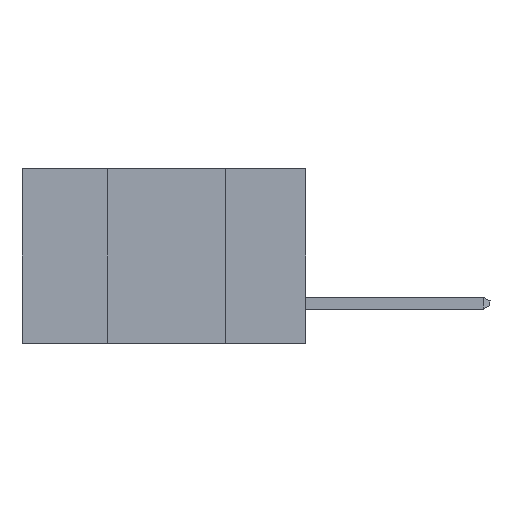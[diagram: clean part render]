
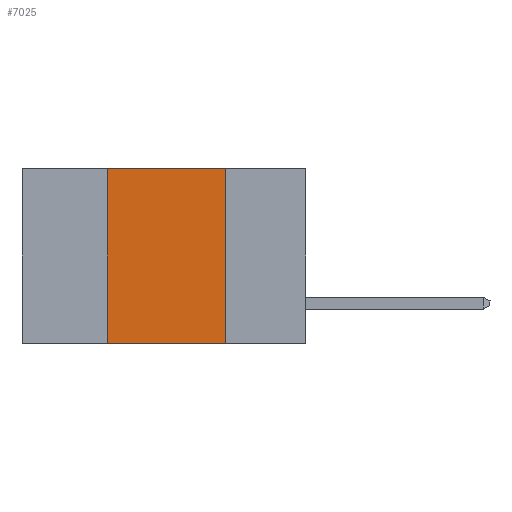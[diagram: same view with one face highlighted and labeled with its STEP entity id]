
A CAD part, left-side view. The second image highlights one B-rep face of the part: STEP entity #7025.
In plain terms, the highlighted planar face has unit normal (-1, 0, 0).
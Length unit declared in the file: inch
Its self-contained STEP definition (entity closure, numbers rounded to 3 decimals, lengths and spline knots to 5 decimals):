
#470 = PLANE ( 'NONE',  #8786 ) ;
#1084 = VERTEX_POINT ( 'NONE', #11166 ) ;
#1556 = DIRECTION ( 'NONE',  ( 0., 0., -1. ) ) ;
#1808 = LINE ( 'NONE', #17013, #13782 ) ;
#2429 = CARTESIAN_POINT ( 'NONE',  ( 0., 0.17, 0. ) ) ;
#3418 = VECTOR ( 'NONE', #16463, 39.37008 ) ;
#4091 = VERTEX_POINT ( 'NONE', #21243 ) ;
#4285 = CARTESIAN_POINT ( 'NONE',  ( 0., 0.6, 0. ) ) ;
#4698 = LINE ( 'NONE', #6714, #3418 ) ;
#6393 = LINE ( 'NONE', #8289, #11943 ) ;
#6714 = CARTESIAN_POINT ( 'NONE',  ( 0., 0.42, -0.37 ) ) ;
#7025 = ADVANCED_FACE ( 'NONE', ( #23585 ), #470, .F. ) ;
#7347 = CARTESIAN_POINT ( 'NONE',  ( 0., 0.42, 0. ) ) ;
#7663 = ORIENTED_EDGE ( 'NONE', *, *, #12597, .F. ) ;
#7950 = VECTOR ( 'NONE', #8448, 39.37008 ) ;
#8289 = CARTESIAN_POINT ( 'NONE',  ( 0., 0.6, 0. ) ) ;
#8448 = DIRECTION ( 'NONE',  ( 0., -1., 0. ) ) ;
#8786 = AXIS2_PLACEMENT_3D ( 'NONE', #4285, #12010, #13796 ) ;
#11166 = CARTESIAN_POINT ( 'NONE',  ( 0., 0.17, -0.37 ) ) ;
#11943 = VECTOR ( 'NONE', #16010, 39.37008 ) ;
#12010 = DIRECTION ( 'NONE',  ( 1., 0., 0. ) ) ;
#12022 = ORIENTED_EDGE ( 'NONE', *, *, #20433, .F. ) ;
#12597 = EDGE_CURVE ( 'NONE', #15292, #1084, #1808, .T. ) ;
#13782 = VECTOR ( 'NONE', #1556, 39.37008 ) ;
#13796 = DIRECTION ( 'NONE',  ( 0., 0., -1. ) ) ;
#15292 = VERTEX_POINT ( 'NONE', #2429 ) ;
#15528 = VERTEX_POINT ( 'NONE', #7347 ) ;
#16010 = DIRECTION ( 'NONE',  ( 0., -1., 0. ) ) ;
#16238 = ORIENTED_EDGE ( 'NONE', *, *, #19672, .F. ) ;
#16285 = LINE ( 'NONE', #22398, #7950 ) ;
#16463 = DIRECTION ( 'NONE',  ( 0., 0., 1. ) ) ;
#17013 = CARTESIAN_POINT ( 'NONE',  ( 0., 0.17, -0.37 ) ) ;
#19102 = ORIENTED_EDGE ( 'NONE', *, *, #21621, .T. ) ;
#19672 = EDGE_CURVE ( 'NONE', #4091, #15528, #4698, .T. ) ;
#20409 = EDGE_LOOP ( 'NONE', ( #7663, #12022, #16238, #19102 ) ) ;
#20433 = EDGE_CURVE ( 'NONE', #15528, #15292, #6393, .T. ) ;
#21243 = CARTESIAN_POINT ( 'NONE',  ( 0., 0.42, -0.37 ) ) ;
#21621 = EDGE_CURVE ( 'NONE', #4091, #1084, #16285, .T. ) ;
#22398 = CARTESIAN_POINT ( 'NONE',  ( 0., 0.6, -0.37 ) ) ;
#23585 = FACE_OUTER_BOUND ( 'NONE', #20409, .T. ) ;
